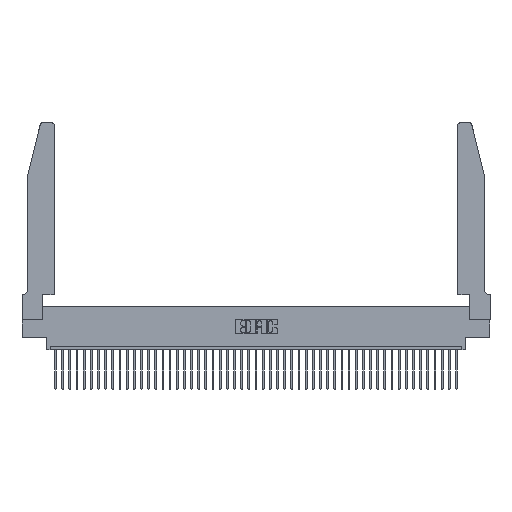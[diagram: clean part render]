
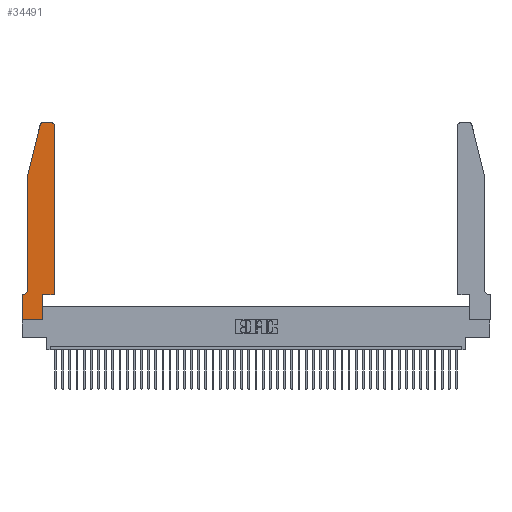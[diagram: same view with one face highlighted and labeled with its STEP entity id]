
A CAD part, top view. The second image highlights one B-rep face of the part: STEP entity #34491.
In plain terms, the highlighted planar face has unit normal (0, 0, 1).
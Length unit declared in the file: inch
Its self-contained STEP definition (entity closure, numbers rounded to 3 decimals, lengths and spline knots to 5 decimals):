
#1393 = VERTEX_POINT ( 'NONE', #11315 ) ;
#1566 = CARTESIAN_POINT ( 'NONE',  ( 0.0755, 0.42, 0.37 ) ) ;
#1580 = CARTESIAN_POINT ( 'NONE',  ( 0.4205, 2.75, 0.37 ) ) ;
#1736 = VECTOR ( 'NONE', #39032, 39.37008 ) ;
#1774 = EDGE_CURVE ( 'NONE', #24338, #15788, #40122, .T. ) ;
#1960 = VERTEX_POINT ( 'NONE', #16445 ) ;
#2485 = CARTESIAN_POINT ( 'NONE',  ( 0.284, 2.72, 0.37 ) ) ;
#3887 = DIRECTION ( 'NONE',  ( -0.239, -0.971, 0. ) ) ;
#4232 = EDGE_CURVE ( 'NONE', #13335, #24338, #43218, .T. ) ;
#5024 = EDGE_CURVE ( 'NONE', #10807, #8868, #22126, .T. ) ;
#5360 = DIRECTION ( 'NONE',  ( 0., -1., 0. ) ) ;
#5414 = CARTESIAN_POINT ( 'NONE',  ( 0.2865, 0.35, 0.37 ) ) ;
#7018 = ORIENTED_EDGE ( 'NONE', *, *, #17579, .T. ) ;
#7799 = ORIENTED_EDGE ( 'NONE', *, *, #37790, .T. ) ;
#8171 = AXIS2_PLACEMENT_3D ( 'NONE', #45803, #35327, #13657 ) ;
#8190 = EDGE_CURVE ( 'NONE', #8868, #31201, #29568, .T. ) ;
#8278 = VERTEX_POINT ( 'NONE', #1566 ) ;
#8484 = DIRECTION ( 'NONE',  ( 1., 0., 0. ) ) ;
#8868 = VERTEX_POINT ( 'NONE', #10448 ) ;
#8885 = VECTOR ( 'NONE', #5360, 39.37008 ) ;
#8888 = DIRECTION ( 'NONE',  ( -1., 0., 0. ) ) ;
#9584 = VERTEX_POINT ( 'NONE', #1580 ) ;
#10448 = CARTESIAN_POINT ( 'NONE',  ( 0.25487, 2.72718, 0.37 ) ) ;
#10807 = VERTEX_POINT ( 'NONE', #44288 ) ;
#11315 = CARTESIAN_POINT ( 'NONE',  ( 0.4505, 2.72, 0.37 ) ) ;
#11532 = CIRCLE ( 'NONE', #13215, 0.07 ) ;
#12315 = CARTESIAN_POINT ( 'NONE',  ( 0.0755, 2., 0.37 ) ) ;
#12998 = AXIS2_PLACEMENT_3D ( 'NONE', #2485, #27204, #13116 ) ;
#13085 = VECTOR ( 'NONE', #28355, 39.37008 ) ;
#13116 = DIRECTION ( 'NONE',  ( 1., 0., 0. ) ) ;
#13215 = AXIS2_PLACEMENT_3D ( 'NONE', #24581, #27885, #31606 ) ;
#13335 = VERTEX_POINT ( 'NONE', #41163 ) ;
#13657 = DIRECTION ( 'NONE',  ( 1., 0., 0. ) ) ;
#14166 = ORIENTED_EDGE ( 'NONE', *, *, #19861, .T. ) ;
#14482 = DIRECTION ( 'NONE',  ( 1., 0., 0. ) ) ;
#14889 = ORIENTED_EDGE ( 'NONE', *, *, #8190, .T. ) ;
#15788 = VERTEX_POINT ( 'NONE', #34864 ) ;
#16445 = CARTESIAN_POINT ( 'NONE',  ( 0.4505, 0.35, 0.37 ) ) ;
#17438 = EDGE_CURVE ( 'NONE', #1393, #9584, #21396, .T. ) ;
#17544 = CARTESIAN_POINT ( 'NONE',  ( 0., 0., 0.37 ) ) ;
#17579 = EDGE_CURVE ( 'NONE', #33447, #1960, #31912, .T. ) ;
#18490 = FACE_OUTER_BOUND ( 'NONE', #45167, .T. ) ;
#19850 = DIRECTION ( 'NONE',  ( 0., 1., 0. ) ) ;
#19861 = EDGE_CURVE ( 'NONE', #31201, #8278, #37135, .T. ) ;
#21274 = EDGE_CURVE ( 'NONE', #8278, #27988, #11532, .T. ) ;
#21396 = CIRCLE ( 'NONE', #8171, 0.03 ) ;
#22126 = CIRCLE ( 'NONE', #12998, 0.03 ) ;
#22463 = VECTOR ( 'NONE', #8484, 39.37008 ) ;
#22535 = VECTOR ( 'NONE', #43996, 39.37008 ) ;
#23023 = CARTESIAN_POINT ( 'NONE',  ( 0.0755, 2., 0.37 ) ) ;
#23361 = LINE ( 'NONE', #36907, #41051 ) ;
#24338 = VERTEX_POINT ( 'NONE', #26659 ) ;
#24356 = ORIENTED_EDGE ( 'NONE', *, *, #26932, .T. ) ;
#24581 = CARTESIAN_POINT ( 'NONE',  ( 0.0055, 0.42, 0.37 ) ) ;
#24675 = CARTESIAN_POINT ( 'NONE',  ( 0., 0.35, 0.37 ) ) ;
#24934 = LINE ( 'NONE', #33475, #1736 ) ;
#24953 = PLANE ( 'NONE',  #45237 ) ;
#25059 = CARTESIAN_POINT ( 'NONE',  ( 0.0755, 2., 0.37 ) ) ;
#25249 = ORIENTED_EDGE ( 'NONE', *, *, #39589, .T. ) ;
#25268 = DIRECTION ( 'NONE',  ( 0., 0., 1. ) ) ;
#25965 = CARTESIAN_POINT ( 'NONE',  ( 0.4505, 0.35, 0.37 ) ) ;
#26659 = CARTESIAN_POINT ( 'NONE',  ( 0., 0., 0.37 ) ) ;
#26932 = EDGE_CURVE ( 'NONE', #1960, #1393, #24934, .T. ) ;
#26945 = CARTESIAN_POINT ( 'NONE',  ( 0., 0., 0.37 ) ) ;
#27204 = DIRECTION ( 'NONE',  ( 0., 0., 1. ) ) ;
#27885 = DIRECTION ( 'NONE',  ( 0., 0., -1. ) ) ;
#27988 = VERTEX_POINT ( 'NONE', #29153 ) ;
#28000 = VECTOR ( 'NONE', #3887, 39.37008 ) ;
#28355 = DIRECTION ( 'NONE',  ( 1., 0., 0. ) ) ;
#29153 = CARTESIAN_POINT ( 'NONE',  ( 0.0055, 0.35, 0.37 ) ) ;
#29568 = LINE ( 'NONE', #25059, #28000 ) ;
#29983 = EDGE_CURVE ( 'NONE', #27988, #13335, #43555, .T. ) ;
#30485 = LINE ( 'NONE', #40668, #38740 ) ;
#30675 = DIRECTION ( 'NONE',  ( 0., -1., 0. ) ) ;
#31201 = VERTEX_POINT ( 'NONE', #12315 ) ;
#31606 = DIRECTION ( 'NONE',  ( -1., 0., 0. ) ) ;
#31912 = LINE ( 'NONE', #25965, #22463 ) ;
#32813 = ORIENTED_EDGE ( 'NONE', *, *, #5024, .T. ) ;
#33447 = VERTEX_POINT ( 'NONE', #5414 ) ;
#33475 = CARTESIAN_POINT ( 'NONE',  ( 0.4505, 0.35, 0.37 ) ) ;
#33870 = VECTOR ( 'NONE', #30675, 39.37008 ) ;
#34491 = ADVANCED_FACE ( 'NONE', ( #18490 ), #24953, .T. ) ;
#34864 = CARTESIAN_POINT ( 'NONE',  ( 0.2865, 0., 0.37 ) ) ;
#35058 = ORIENTED_EDGE ( 'NONE', *, *, #21274, .T. ) ;
#35327 = DIRECTION ( 'NONE',  ( 0., 0., 1. ) ) ;
#36759 = ORIENTED_EDGE ( 'NONE', *, *, #29983, .T. ) ;
#36902 = CARTESIAN_POINT ( 'NONE',  ( 0.0755, 0.35, 0.37 ) ) ;
#36907 = CARTESIAN_POINT ( 'NONE',  ( 0.2605, 2.75, 0.37 ) ) ;
#37135 = LINE ( 'NONE', #23023, #8885 ) ;
#37790 = EDGE_CURVE ( 'NONE', #9584, #10807, #23361, .T. ) ;
#38740 = VECTOR ( 'NONE', #19850, 39.37008 ) ;
#39032 = DIRECTION ( 'NONE',  ( 0., 1., 0. ) ) ;
#39589 = EDGE_CURVE ( 'NONE', #15788, #33447, #30485, .T. ) ;
#39914 = ORIENTED_EDGE ( 'NONE', *, *, #1774, .T. ) ;
#40122 = LINE ( 'NONE', #17544, #13085 ) ;
#40668 = CARTESIAN_POINT ( 'NONE',  ( 0.2865, 0.35, 0.37 ) ) ;
#41051 = VECTOR ( 'NONE', #8888, 39.37008 ) ;
#41163 = CARTESIAN_POINT ( 'NONE',  ( 0., 0.35, 0.37 ) ) ;
#43218 = LINE ( 'NONE', #26945, #33870 ) ;
#43344 = ORIENTED_EDGE ( 'NONE', *, *, #17438, .T. ) ;
#43555 = LINE ( 'NONE', #36902, #22535 ) ;
#43996 = DIRECTION ( 'NONE',  ( -1., 0., 0. ) ) ;
#44288 = CARTESIAN_POINT ( 'NONE',  ( 0.284, 2.75, 0.37 ) ) ;
#44573 = ORIENTED_EDGE ( 'NONE', *, *, #4232, .T. ) ;
#45167 = EDGE_LOOP ( 'NONE', ( #7799, #32813, #14889, #14166, #35058, #36759, #44573, #39914, #25249, #7018, #24356, #43344 ) ) ;
#45237 = AXIS2_PLACEMENT_3D ( 'NONE', #24675, #25268, #14482 ) ;
#45803 = CARTESIAN_POINT ( 'NONE',  ( 0.4205, 2.72, 0.37 ) ) ;
